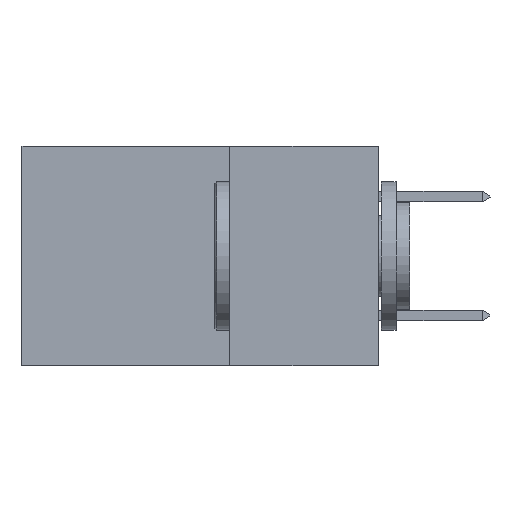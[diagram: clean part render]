
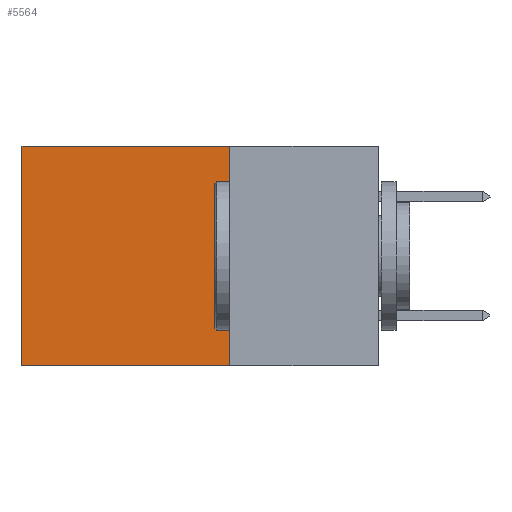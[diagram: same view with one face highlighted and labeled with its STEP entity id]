
A CAD part, left-side view. The second image highlights one B-rep face of the part: STEP entity #5564.
In plain terms, the highlighted planar face has unit normal (-1, 0, 0).
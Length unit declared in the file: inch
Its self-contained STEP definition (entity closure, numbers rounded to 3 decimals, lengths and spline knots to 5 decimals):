
#1914 = DIRECTION ( 'NONE',  ( 0., 0., -1. ) ) ;
#2141 = ORIENTED_EDGE ( 'NONE', *, *, #16521, .F. ) ;
#3326 = LINE ( 'NONE', #13216, #24051 ) ;
#3800 = VERTEX_POINT ( 'NONE', #8778 ) ;
#4069 = VECTOR ( 'NONE', #19660, 39.37008 ) ;
#4360 = FACE_OUTER_BOUND ( 'NONE', #10717, .T. ) ;
#4732 = VECTOR ( 'NONE', #14068, 39.37008 ) ;
#5564 = ADVANCED_FACE ( 'NONE', ( #4360 ), #21888, .F. ) ;
#5570 = EDGE_CURVE ( 'NONE', #3800, #23457, #10873, .T. ) ;
#5870 = CARTESIAN_POINT ( 'NONE',  ( 0.298, 0.25, 0. ) ) ;
#7673 = DIRECTION ( 'NONE',  ( 0., 0., -1. ) ) ;
#8466 = CARTESIAN_POINT ( 'NONE',  ( 0.298, 0.25, 0. ) ) ;
#8742 = LINE ( 'NONE', #15547, #4732 ) ;
#8778 = CARTESIAN_POINT ( 'NONE',  ( 0.298, 0.25, 0. ) ) ;
#9874 = CARTESIAN_POINT ( 'NONE',  ( 0.298, 0.6, -0.37 ) ) ;
#10717 = EDGE_LOOP ( 'NONE', ( #12809, #2141, #20043, #16655 ) ) ;
#10873 = LINE ( 'NONE', #19919, #4069 ) ;
#12809 = ORIENTED_EDGE ( 'NONE', *, *, #13261, .T. ) ;
#12873 = DIRECTION ( 'NONE',  ( 0., 0., -1. ) ) ;
#13216 = CARTESIAN_POINT ( 'NONE',  ( 0.298, 0.6, 0. ) ) ;
#13261 = EDGE_CURVE ( 'NONE', #23457, #25254, #3326, .T. ) ;
#13726 = VECTOR ( 'NONE', #12873, 39.37008 ) ;
#14068 = DIRECTION ( 'NONE',  ( 0., 1., 0. ) ) ;
#15547 = CARTESIAN_POINT ( 'NONE',  ( 0.298, 0.25, -0.37 ) ) ;
#16521 = EDGE_CURVE ( 'NONE', #17577, #25254, #8742, .T. ) ;
#16655 = ORIENTED_EDGE ( 'NONE', *, *, #5570, .T. ) ;
#17577 = VERTEX_POINT ( 'NONE', #20460 ) ;
#17614 = EDGE_CURVE ( 'NONE', #3800, #17577, #23634, .T. ) ;
#17893 = CARTESIAN_POINT ( 'NONE',  ( 0.298, 0.6, 0. ) ) ;
#19660 = DIRECTION ( 'NONE',  ( 0., 1., 0. ) ) ;
#19919 = CARTESIAN_POINT ( 'NONE',  ( 0.298, 0.25, 0. ) ) ;
#20043 = ORIENTED_EDGE ( 'NONE', *, *, #17614, .F. ) ;
#20460 = CARTESIAN_POINT ( 'NONE',  ( 0.298, 0.25, -0.37 ) ) ;
#21720 = DIRECTION ( 'NONE',  ( 1., 0., 0. ) ) ;
#21888 = PLANE ( 'NONE',  #23167 ) ;
#23167 = AXIS2_PLACEMENT_3D ( 'NONE', #5870, #21720, #7673 ) ;
#23457 = VERTEX_POINT ( 'NONE', #17893 ) ;
#23634 = LINE ( 'NONE', #8466, #13726 ) ;
#24051 = VECTOR ( 'NONE', #1914, 39.37008 ) ;
#25254 = VERTEX_POINT ( 'NONE', #9874 ) ;
